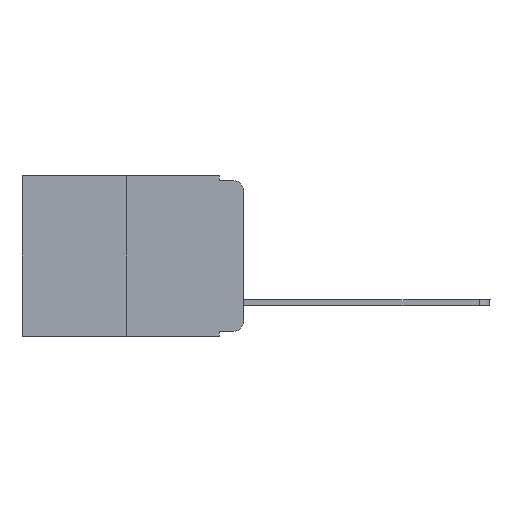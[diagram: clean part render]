
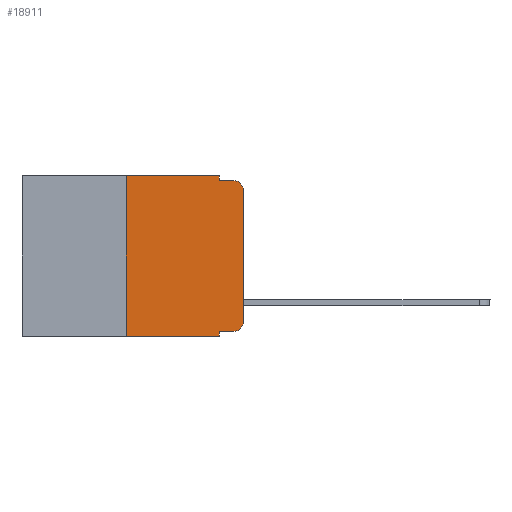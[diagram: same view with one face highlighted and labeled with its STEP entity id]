
A CAD part, left-side view. The second image highlights one B-rep face of the part: STEP entity #18911.
In plain terms, the highlighted planar face has unit normal (-1, 0, 0).
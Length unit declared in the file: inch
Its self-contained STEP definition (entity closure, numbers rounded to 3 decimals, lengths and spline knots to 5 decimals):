
#151 = DIRECTION ( 'NONE',  ( -1., 0., 0. ) ) ;
#154 = ORIENTED_EDGE ( 'NONE', *, *, #7761, .F. ) ;
#242 = EDGE_CURVE ( 'NONE', #1463, #1744, #6692, .T. ) ;
#372 = ORIENTED_EDGE ( 'NONE', *, *, #8672, .F. ) ;
#403 = DIRECTION ( 'NONE',  ( 0., 0., -1. ) ) ;
#444 = DIRECTION ( 'NONE',  ( 0., -1., 0. ) ) ;
#834 = CARTESIAN_POINT ( 'NONE',  ( 0., 0.051, 0. ) ) ;
#937 = LINE ( 'NONE', #834, #19724 ) ;
#1282 = ORIENTED_EDGE ( 'NONE', *, *, #15228, .F. ) ;
#1463 = VERTEX_POINT ( 'NONE', #17087 ) ;
#1619 = VECTOR ( 'NONE', #11989, 39.37008 ) ;
#1621 = EDGE_CURVE ( 'NONE', #5924, #11238, #8068, .T. ) ;
#1696 = CIRCLE ( 'NONE', #17688, 0.02 ) ;
#1744 = VERTEX_POINT ( 'NONE', #14984 ) ;
#1801 = ORIENTED_EDGE ( 'NONE', *, *, #12905, .F. ) ;
#1913 = DIRECTION ( 'NONE',  ( -1., 0., 0. ) ) ;
#2391 = CARTESIAN_POINT ( 'NONE',  ( 0., 0.051, 0. ) ) ;
#3034 = LINE ( 'NONE', #9424, #10609 ) ;
#3281 = DIRECTION ( 'NONE',  ( 1., 0., 0. ) ) ;
#3374 = VERTEX_POINT ( 'NONE', #14572 ) ;
#3507 = ORIENTED_EDGE ( 'NONE', *, *, #19008, .T. ) ;
#3591 = DIRECTION ( 'NONE',  ( 0., -1., 0. ) ) ;
#3958 = CARTESIAN_POINT ( 'NONE',  ( 0., 0., -0.03 ) ) ;
#4484 = CARTESIAN_POINT ( 'NONE',  ( 0., 0.02, -0.03 ) ) ;
#5270 = LINE ( 'NONE', #14591, #16310 ) ;
#5328 = ORIENTED_EDGE ( 'NONE', *, *, #242, .F. ) ;
#5428 = VERTEX_POINT ( 'NONE', #2391 ) ;
#5678 = CARTESIAN_POINT ( 'NONE',  ( 0., 0., -0.313 ) ) ;
#5786 = CARTESIAN_POINT ( 'NONE',  ( 0., 0.473, -0.343 ) ) ;
#5834 = EDGE_CURVE ( 'NONE', #19173, #6997, #5270, .T. ) ;
#5924 = VERTEX_POINT ( 'NONE', #13835 ) ;
#6543 = CARTESIAN_POINT ( 'NONE',  ( 0., 0.02, -0.313 ) ) ;
#6692 = LINE ( 'NONE', #10881, #9767 ) ;
#6802 = EDGE_CURVE ( 'NONE', #1463, #15185, #17897, .T. ) ;
#6997 = VERTEX_POINT ( 'NONE', #3958 ) ;
#7052 = CARTESIAN_POINT ( 'NONE',  ( 0., 0.473, 0. ) ) ;
#7761 = EDGE_CURVE ( 'NONE', #5428, #3374, #3034, .T. ) ;
#8068 = LINE ( 'NONE', #14180, #12963 ) ;
#8560 = DIRECTION ( 'NONE',  ( 0., 0., -1. ) ) ;
#8635 = DIRECTION ( 'NONE',  ( 0., -1., 0. ) ) ;
#8672 = EDGE_CURVE ( 'NONE', #1744, #5428, #11741, .T. ) ;
#9191 = FACE_OUTER_BOUND ( 'NONE', #16454, .T. ) ;
#9285 = ORIENTED_EDGE ( 'NONE', *, *, #1621, .T. ) ;
#9424 = CARTESIAN_POINT ( 'NONE',  ( 0., 0.051, 0. ) ) ;
#9560 = CARTESIAN_POINT ( 'NONE',  ( 0., 0.02, -0.01 ) ) ;
#9767 = VECTOR ( 'NONE', #18804, 39.37008 ) ;
#10559 = VERTEX_POINT ( 'NONE', #9560 ) ;
#10609 = VECTOR ( 'NONE', #10822, 39.37008 ) ;
#10822 = DIRECTION ( 'NONE',  ( 0., 0., -1. ) ) ;
#10881 = CARTESIAN_POINT ( 'NONE',  ( 0., 0.25, 0. ) ) ;
#11238 = VERTEX_POINT ( 'NONE', #18142 ) ;
#11251 = AXIS2_PLACEMENT_3D ( 'NONE', #6543, #1913, #403 ) ;
#11741 = LINE ( 'NONE', #7052, #17680 ) ;
#11989 = DIRECTION ( 'NONE',  ( 0., -1., 0. ) ) ;
#12390 = DIRECTION ( 'NONE',  ( 0., 0., -1. ) ) ;
#12504 = CARTESIAN_POINT ( 'NONE',  ( 0., 0.051, -0.01 ) ) ;
#12905 = EDGE_CURVE ( 'NONE', #3374, #10559, #17306, .T. ) ;
#12963 = VECTOR ( 'NONE', #444, 39.37008 ) ;
#13176 = CIRCLE ( 'NONE', #11251, 0.02 ) ;
#13531 = AXIS2_PLACEMENT_3D ( 'NONE', #19728, #3281, #15396 ) ;
#13627 = ORIENTED_EDGE ( 'NONE', *, *, #18075, .T. ) ;
#13835 = CARTESIAN_POINT ( 'NONE',  ( 0., 0.051, -0.333 ) ) ;
#14180 = CARTESIAN_POINT ( 'NONE',  ( 0., 0.051, -0.333 ) ) ;
#14368 = CARTESIAN_POINT ( 'NONE',  ( 0., 0.051, -0.343 ) ) ;
#14378 = DIRECTION ( 'NONE',  ( 0., 0., 1. ) ) ;
#14572 = CARTESIAN_POINT ( 'NONE',  ( 0., 0.051, -0.01 ) ) ;
#14591 = CARTESIAN_POINT ( 'NONE',  ( 0., 0., 0. ) ) ;
#14945 = ORIENTED_EDGE ( 'NONE', *, *, #6802, .T. ) ;
#14984 = CARTESIAN_POINT ( 'NONE',  ( 0., 0.25, 0. ) ) ;
#15185 = VERTEX_POINT ( 'NONE', #14368 ) ;
#15228 = EDGE_CURVE ( 'NONE', #5924, #15185, #937, .T. ) ;
#15396 = DIRECTION ( 'NONE',  ( 0., 0., -1. ) ) ;
#15851 = ORIENTED_EDGE ( 'NONE', *, *, #5834, .T. ) ;
#16310 = VECTOR ( 'NONE', #14378, 39.37008 ) ;
#16454 = EDGE_LOOP ( 'NONE', ( #15851, #3507, #1801, #154, #372, #5328, #14945, #1282, #9285, #13627 ) ) ;
#17087 = CARTESIAN_POINT ( 'NONE',  ( 0., 0.25, -0.343 ) ) ;
#17117 = VECTOR ( 'NONE', #3591, 39.37008 ) ;
#17306 = LINE ( 'NONE', #12504, #17117 ) ;
#17680 = VECTOR ( 'NONE', #8635, 39.37008 ) ;
#17688 = AXIS2_PLACEMENT_3D ( 'NONE', #4484, #151, #12390 ) ;
#17897 = LINE ( 'NONE', #5786, #1619 ) ;
#18075 = EDGE_CURVE ( 'NONE', #11238, #19173, #13176, .T. ) ;
#18142 = CARTESIAN_POINT ( 'NONE',  ( 0., 0.02, -0.333 ) ) ;
#18593 = PLANE ( 'NONE',  #13531 ) ;
#18804 = DIRECTION ( 'NONE',  ( 0., 0., 1. ) ) ;
#18911 = ADVANCED_FACE ( 'NONE', ( #9191 ), #18593, .F. ) ;
#19008 = EDGE_CURVE ( 'NONE', #6997, #10559, #1696, .T. ) ;
#19173 = VERTEX_POINT ( 'NONE', #5678 ) ;
#19724 = VECTOR ( 'NONE', #8560, 39.37008 ) ;
#19728 = CARTESIAN_POINT ( 'NONE',  ( 0., 0.473, 0. ) ) ;
